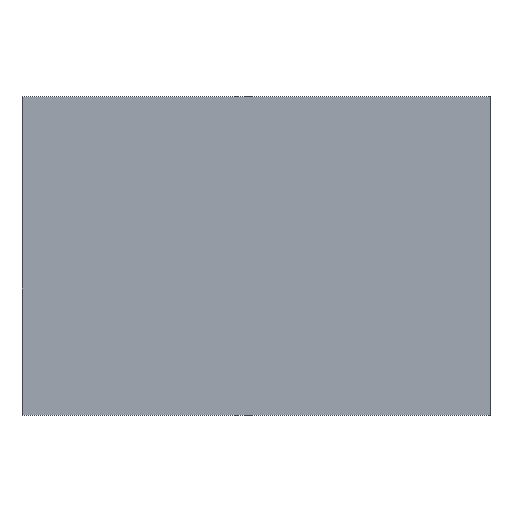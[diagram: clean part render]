
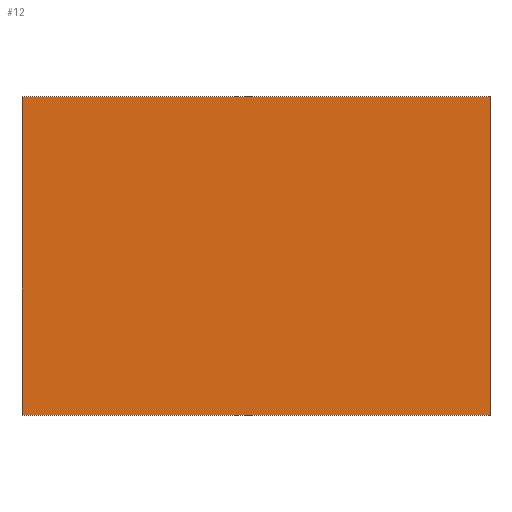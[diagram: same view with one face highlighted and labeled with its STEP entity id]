
A CAD part, top view. The second image highlights one B-rep face of the part: STEP entity #12.
In plain terms, the highlighted planar face has unit normal (0, 0, 1).
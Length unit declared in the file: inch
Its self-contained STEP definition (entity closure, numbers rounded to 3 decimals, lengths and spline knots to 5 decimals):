
#2 = CARTESIAN_POINT ( 'NONE',  ( -0.625, -0.425, 0.1 ) ) ;
#12 = ADVANCED_FACE ( 'NONE', ( #45 ), #170, .F. ) ;
#39 = EDGE_CURVE ( 'NONE', #300, #322, #274, .T. ) ;
#45 = FACE_OUTER_BOUND ( 'NONE', #242, .T. ) ;
#49 = EDGE_CURVE ( 'NONE', #322, #83, #275, .T. ) ;
#83 = VERTEX_POINT ( 'NONE', #327 ) ;
#89 = VECTOR ( 'NONE', #160, 39.37008 ) ;
#110 = ORIENTED_EDGE ( 'NONE', *, *, #39, .T. ) ;
#116 = CARTESIAN_POINT ( 'NONE',  ( 0., 0., 0.1 ) ) ;
#143 = DIRECTION ( 'NONE',  ( 0., 1., 0. ) ) ;
#144 = LINE ( 'NONE', #335, #89 ) ;
#160 = DIRECTION ( 'NONE',  ( -1., 0., 0. ) ) ;
#170 = PLANE ( 'NONE',  #179 ) ;
#179 = AXIS2_PLACEMENT_3D ( 'NONE', #116, #247, #296 ) ;
#195 = VECTOR ( 'NONE', #143, 39.37008 ) ;
#214 = CARTESIAN_POINT ( 'NONE',  ( 0.625, -0.425, 0.1 ) ) ;
#226 = VECTOR ( 'NONE', #298, 39.37008 ) ;
#229 = EDGE_CURVE ( 'NONE', #264, #300, #250, .T. ) ;
#232 = ORIENTED_EDGE ( 'NONE', *, *, #49, .T. ) ;
#238 = DIRECTION ( 'NONE',  ( 0., -1., 0. ) ) ;
#240 = CARTESIAN_POINT ( 'NONE',  ( -0.625, -0.425, 0.1 ) ) ;
#242 = EDGE_LOOP ( 'NONE', ( #232, #306, #270, #110 ) ) ;
#247 = DIRECTION ( 'NONE',  ( 0., 0., -1. ) ) ;
#250 = LINE ( 'NONE', #240, #319 ) ;
#260 = CARTESIAN_POINT ( 'NONE',  ( -0.625, -0.425, 0.1 ) ) ;
#264 = VERTEX_POINT ( 'NONE', #284 ) ;
#270 = ORIENTED_EDGE ( 'NONE', *, *, #229, .T. ) ;
#274 = LINE ( 'NONE', #2, #226 ) ;
#275 = LINE ( 'NONE', #295, #195 ) ;
#284 = CARTESIAN_POINT ( 'NONE',  ( -0.625, 0.425, 0.1 ) ) ;
#295 = CARTESIAN_POINT ( 'NONE',  ( 0.625, -0.425, 0.1 ) ) ;
#296 = DIRECTION ( 'NONE',  ( -1., 0., 0. ) ) ;
#298 = DIRECTION ( 'NONE',  ( 1., 0., 0. ) ) ;
#300 = VERTEX_POINT ( 'NONE', #260 ) ;
#304 = EDGE_CURVE ( 'NONE', #83, #264, #144, .T. ) ;
#306 = ORIENTED_EDGE ( 'NONE', *, *, #304, .T. ) ;
#319 = VECTOR ( 'NONE', #238, 39.37008 ) ;
#322 = VERTEX_POINT ( 'NONE', #214 ) ;
#327 = CARTESIAN_POINT ( 'NONE',  ( 0.625, 0.425, 0.1 ) ) ;
#335 = CARTESIAN_POINT ( 'NONE',  ( -0.625, 0.425, 0.1 ) ) ;
